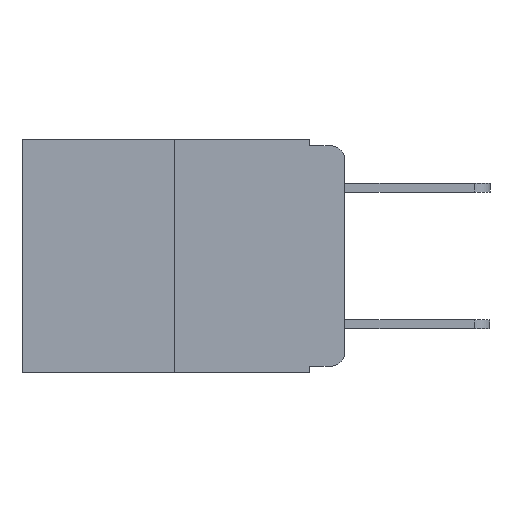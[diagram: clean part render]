
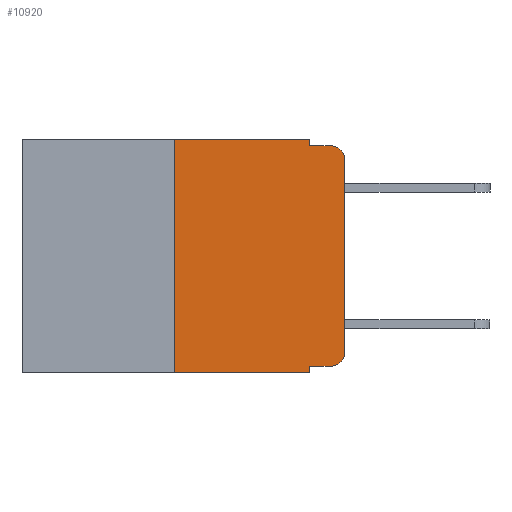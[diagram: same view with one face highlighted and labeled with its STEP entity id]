
A CAD part, left-side view. The second image highlights one B-rep face of the part: STEP entity #10920.
In plain terms, the highlighted planar face has unit normal (-1, 0, 0).
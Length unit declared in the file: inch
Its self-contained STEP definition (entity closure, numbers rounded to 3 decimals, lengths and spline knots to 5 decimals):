
#256 = EDGE_CURVE ( 'NONE', #3430, #2351, #19089, .T. ) ;
#341 = DIRECTION ( 'NONE',  ( 0., -1., 0. ) ) ;
#1000 = LINE ( 'NONE', #13159, #19418 ) ;
#1281 = PLANE ( 'NONE',  #9674 ) ;
#1684 = CARTESIAN_POINT ( 'NONE',  ( 0., 0.473, -0.343 ) ) ;
#1994 = EDGE_CURVE ( 'NONE', #2813, #22535, #7803, .T. ) ;
#2351 = VERTEX_POINT ( 'NONE', #13136 ) ;
#2441 = VECTOR ( 'NONE', #341, 39.37008 ) ;
#2813 = VERTEX_POINT ( 'NONE', #16270 ) ;
#2857 = EDGE_CURVE ( 'NONE', #20318, #5480, #14047, .T. ) ;
#3338 = VECTOR ( 'NONE', #6090, 39.37008 ) ;
#3359 = CARTESIAN_POINT ( 'NONE',  ( 0., 0.051, 0. ) ) ;
#3430 = VERTEX_POINT ( 'NONE', #11315 ) ;
#3609 = CARTESIAN_POINT ( 'NONE',  ( 0., 0.02, -0.03 ) ) ;
#3788 = DIRECTION ( 'NONE',  ( 0., 0., -1. ) ) ;
#3881 = ORIENTED_EDGE ( 'NONE', *, *, #15189, .F. ) ;
#3923 = LINE ( 'NONE', #22199, #3338 ) ;
#4424 = LINE ( 'NONE', #9788, #22628 ) ;
#4623 = VECTOR ( 'NONE', #14599, 39.37008 ) ;
#4815 = ORIENTED_EDGE ( 'NONE', *, *, #5279, .T. ) ;
#5052 = CARTESIAN_POINT ( 'NONE',  ( 0., 0.473, 0. ) ) ;
#5165 = DIRECTION ( 'NONE',  ( -1., 0., 0. ) ) ;
#5279 = EDGE_CURVE ( 'NONE', #5532, #3430, #3923, .T. ) ;
#5480 = VERTEX_POINT ( 'NONE', #3359 ) ;
#5529 = CARTESIAN_POINT ( 'NONE',  ( 0., 0.473, 0. ) ) ;
#5532 = VERTEX_POINT ( 'NONE', #11187 ) ;
#6090 = DIRECTION ( 'NONE',  ( 0., 0., 1. ) ) ;
#6108 = VECTOR ( 'NONE', #18511, 39.37008 ) ;
#6229 = CARTESIAN_POINT ( 'NONE',  ( 0., 0.25, 0. ) ) ;
#6397 = ORIENTED_EDGE ( 'NONE', *, *, #2857, .F. ) ;
#6895 = DIRECTION ( 'NONE',  ( 1., 0., 0. ) ) ;
#7803 = LINE ( 'NONE', #19031, #17090 ) ;
#7861 = ORIENTED_EDGE ( 'NONE', *, *, #12157, .T. ) ;
#7882 = ORIENTED_EDGE ( 'NONE', *, *, #1994, .F. ) ;
#8658 = EDGE_CURVE ( 'NONE', #11122, #22535, #12260, .T. ) ;
#9146 = CARTESIAN_POINT ( 'NONE',  ( 0., 0.02, -0.313 ) ) ;
#9364 = EDGE_CURVE ( 'NONE', #11122, #20318, #9775, .T. ) ;
#9615 = CARTESIAN_POINT ( 'NONE',  ( 0., 0.051, -0.333 ) ) ;
#9674 = AXIS2_PLACEMENT_3D ( 'NONE', #5052, #6895, #19137 ) ;
#9758 = DIRECTION ( 'NONE',  ( 0., 0., -1. ) ) ;
#9775 = LINE ( 'NONE', #6229, #6108 ) ;
#9788 = CARTESIAN_POINT ( 'NONE',  ( 0., 0.051, -0.01 ) ) ;
#10033 = ORIENTED_EDGE ( 'NONE', *, *, #17525, .F. ) ;
#10301 = EDGE_LOOP ( 'NONE', ( #4815, #14746, #10033, #3881, #6397, #14835, #17435, #7882, #19326, #7861 ) ) ;
#10344 = CIRCLE ( 'NONE', #13750, 0.02 ) ;
#10687 = AXIS2_PLACEMENT_3D ( 'NONE', #3609, #5165, #3788 ) ;
#10920 = ADVANCED_FACE ( 'NONE', ( #18672 ), #1281, .F. ) ;
#10947 = DIRECTION ( 'NONE',  ( 0., 0., -1. ) ) ;
#11122 = VERTEX_POINT ( 'NONE', #21492 ) ;
#11187 = CARTESIAN_POINT ( 'NONE',  ( 0., 0., -0.313 ) ) ;
#11188 = VECTOR ( 'NONE', #22492, 39.37008 ) ;
#11315 = CARTESIAN_POINT ( 'NONE',  ( 0., 0., -0.03 ) ) ;
#11572 = CARTESIAN_POINT ( 'NONE',  ( 0., 0.051, -0.01 ) ) ;
#12046 = CARTESIAN_POINT ( 'NONE',  ( 0., 0.02, -0.333 ) ) ;
#12057 = LINE ( 'NONE', #9615, #2441 ) ;
#12157 = EDGE_CURVE ( 'NONE', #18270, #5532, #10344, .T. ) ;
#12260 = LINE ( 'NONE', #1684, #11188 ) ;
#13136 = CARTESIAN_POINT ( 'NONE',  ( 0., 0.02, -0.01 ) ) ;
#13159 = CARTESIAN_POINT ( 'NONE',  ( 0., 0.051, 0. ) ) ;
#13482 = CARTESIAN_POINT ( 'NONE',  ( 0., 0.25, 0. ) ) ;
#13750 = AXIS2_PLACEMENT_3D ( 'NONE', #9146, #21337, #10947 ) ;
#14047 = LINE ( 'NONE', #5529, #4623 ) ;
#14599 = DIRECTION ( 'NONE',  ( 0., -1., 0. ) ) ;
#14746 = ORIENTED_EDGE ( 'NONE', *, *, #256, .T. ) ;
#14835 = ORIENTED_EDGE ( 'NONE', *, *, #9364, .F. ) ;
#15189 = EDGE_CURVE ( 'NONE', #5480, #21530, #1000, .T. ) ;
#16270 = CARTESIAN_POINT ( 'NONE',  ( 0., 0.051, -0.333 ) ) ;
#17090 = VECTOR ( 'NONE', #20221, 39.37008 ) ;
#17138 = DIRECTION ( 'NONE',  ( 0., -1., 0. ) ) ;
#17435 = ORIENTED_EDGE ( 'NONE', *, *, #8658, .T. ) ;
#17525 = EDGE_CURVE ( 'NONE', #21530, #2351, #4424, .T. ) ;
#17966 = EDGE_CURVE ( 'NONE', #2813, #18270, #12057, .T. ) ;
#18270 = VERTEX_POINT ( 'NONE', #12046 ) ;
#18511 = DIRECTION ( 'NONE',  ( 0., 0., 1. ) ) ;
#18672 = FACE_OUTER_BOUND ( 'NONE', #10301, .T. ) ;
#19031 = CARTESIAN_POINT ( 'NONE',  ( 0., 0.051, 0. ) ) ;
#19089 = CIRCLE ( 'NONE', #10687, 0.02 ) ;
#19137 = DIRECTION ( 'NONE',  ( 0., 0., -1. ) ) ;
#19326 = ORIENTED_EDGE ( 'NONE', *, *, #17966, .T. ) ;
#19418 = VECTOR ( 'NONE', #9758, 39.37008 ) ;
#20221 = DIRECTION ( 'NONE',  ( 0., 0., -1. ) ) ;
#20318 = VERTEX_POINT ( 'NONE', #13482 ) ;
#21337 = DIRECTION ( 'NONE',  ( -1., 0., 0. ) ) ;
#21492 = CARTESIAN_POINT ( 'NONE',  ( 0., 0.25, -0.343 ) ) ;
#21530 = VERTEX_POINT ( 'NONE', #11572 ) ;
#22199 = CARTESIAN_POINT ( 'NONE',  ( 0., 0., 0. ) ) ;
#22492 = DIRECTION ( 'NONE',  ( 0., -1., 0. ) ) ;
#22535 = VERTEX_POINT ( 'NONE', #22934 ) ;
#22628 = VECTOR ( 'NONE', #17138, 39.37008 ) ;
#22934 = CARTESIAN_POINT ( 'NONE',  ( 0., 0.051, -0.343 ) ) ;
